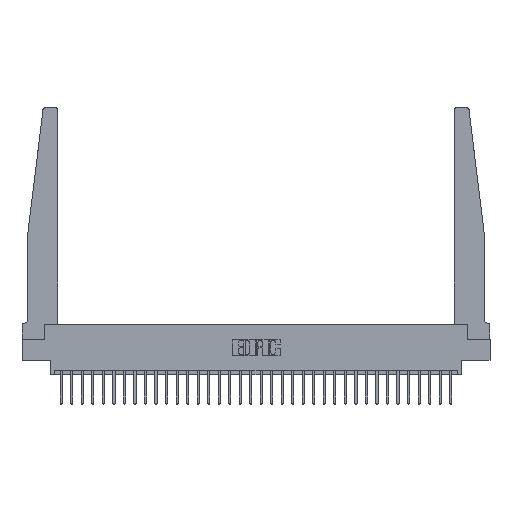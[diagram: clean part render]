
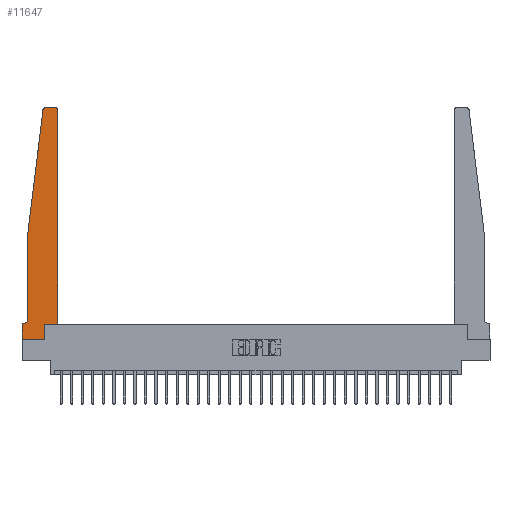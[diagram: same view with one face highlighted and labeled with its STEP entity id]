
A CAD part, top view. The second image highlights one B-rep face of the part: STEP entity #11647.
In plain terms, the highlighted planar face has unit normal (0, 0, 1).
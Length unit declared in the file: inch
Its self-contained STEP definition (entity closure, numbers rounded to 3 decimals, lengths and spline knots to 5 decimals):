
#126 = FACE_OUTER_BOUND ( 'NONE', #1738, .T. ) ;
#573 = DIRECTION ( 'NONE',  ( 1., 0., 0. ) ) ;
#765 = DIRECTION ( 'NONE',  ( -1., 0., 0. ) ) ;
#1738 = EDGE_LOOP ( 'NONE', ( #14604, #15511, #18956, #3326, #2910, #1840, #23805, #4217, #19365, #21651, #21464, #3063 ) ) ;
#1840 = ORIENTED_EDGE ( 'NONE', *, *, #16754, .T. ) ;
#2118 = CARTESIAN_POINT ( 'NONE',  ( 0.25, 2.75, 0.37 ) ) ;
#2347 = VECTOR ( 'NONE', #26820, 39.37008 ) ;
#2727 = VECTOR ( 'NONE', #13173, 39.37008 ) ;
#2849 = VERTEX_POINT ( 'NONE', #7482 ) ;
#2910 = ORIENTED_EDGE ( 'NONE', *, *, #19594, .T. ) ;
#3063 = ORIENTED_EDGE ( 'NONE', *, *, #20286, .T. ) ;
#3131 = VERTEX_POINT ( 'NONE', #7297 ) ;
#3290 = CARTESIAN_POINT ( 'NONE',  ( 0., 0., 0.37 ) ) ;
#3326 = ORIENTED_EDGE ( 'NONE', *, *, #26223, .T. ) ;
#3501 = VERTEX_POINT ( 'NONE', #27071 ) ;
#3511 = VECTOR ( 'NONE', #28980, 39.37008 ) ;
#3869 = DIRECTION ( 'NONE',  ( 1., 0., 0. ) ) ;
#4111 = LINE ( 'NONE', #18639, #15181 ) ;
#4217 = ORIENTED_EDGE ( 'NONE', *, *, #26971, .T. ) ;
#4443 = LINE ( 'NONE', #2118, #30245 ) ;
#5444 = CARTESIAN_POINT ( 'NONE',  ( 0.27653, 2.75, 0.37 ) ) ;
#5943 = LINE ( 'NONE', #15333, #2347 ) ;
#6011 = VERTEX_POINT ( 'NONE', #18988 ) ;
#7297 = CARTESIAN_POINT ( 'NONE',  ( 0.425, 0.18, 0.37 ) ) ;
#7482 = CARTESIAN_POINT ( 'NONE',  ( 0.2605, 0.18, 0.37 ) ) ;
#9328 = CARTESIAN_POINT ( 'NONE',  ( 0., 0.1875, 0.37 ) ) ;
#9490 = CARTESIAN_POINT ( 'NONE',  ( 0., 0.1875, 0.37 ) ) ;
#9556 = CIRCLE ( 'NONE', #13543, 0.03 ) ;
#9811 = LINE ( 'NONE', #11715, #11964 ) ;
#10346 = LINE ( 'NONE', #25306, #2727 ) ;
#10511 = DIRECTION ( 'NONE',  ( 1., 0., 0. ) ) ;
#10516 = VERTEX_POINT ( 'NONE', #26833 ) ;
#11459 = EDGE_CURVE ( 'NONE', #6011, #2849, #19803, .T. ) ;
#11647 = ADVANCED_FACE ( 'NONE', ( #126 ), #14461, .T. ) ;
#11715 = CARTESIAN_POINT ( 'NONE',  ( 0.065, 1.25, 0.37 ) ) ;
#11759 = VECTOR ( 'NONE', #573, 39.37008 ) ;
#11964 = VECTOR ( 'NONE', #23856, 39.37008 ) ;
#12364 = LINE ( 'NONE', #19540, #3511 ) ;
#12996 = VERTEX_POINT ( 'NONE', #14139 ) ;
#13173 = DIRECTION ( 'NONE',  ( 0., -1., 0. ) ) ;
#13422 = EDGE_CURVE ( 'NONE', #3131, #24890, #4111, .T. ) ;
#13543 = AXIS2_PLACEMENT_3D ( 'NONE', #29840, #24900, #3869 ) ;
#13636 = DIRECTION ( 'NONE',  ( 0., 1., 0. ) ) ;
#14139 = CARTESIAN_POINT ( 'NONE',  ( 0.395, 2.75, 0.37 ) ) ;
#14255 = AXIS2_PLACEMENT_3D ( 'NONE', #22997, #15521, #10511 ) ;
#14461 = PLANE ( 'NONE',  #19592 ) ;
#14604 = ORIENTED_EDGE ( 'NONE', *, *, #30408, .T. ) ;
#14779 = LINE ( 'NONE', #17417, #11759 ) ;
#14831 = EDGE_CURVE ( 'NONE', #21649, #27962, #5943, .T. ) ;
#15181 = VECTOR ( 'NONE', #13636, 39.37008 ) ;
#15333 = CARTESIAN_POINT ( 'NONE',  ( 0., 0., 0.37 ) ) ;
#15511 = ORIENTED_EDGE ( 'NONE', *, *, #27499, .T. ) ;
#15521 = DIRECTION ( 'NONE',  ( 0., 0., 1. ) ) ;
#16754 = EDGE_CURVE ( 'NONE', #3501, #21649, #17145, .T. ) ;
#17145 = LINE ( 'NONE', #21131, #18878 ) ;
#17417 = CARTESIAN_POINT ( 'NONE',  ( 0., 0., 0.37 ) ) ;
#18247 = CIRCLE ( 'NONE', #14255, 0.03 ) ;
#18352 = VERTEX_POINT ( 'NONE', #23576 ) ;
#18365 = EDGE_CURVE ( 'NONE', #10516, #26652, #9811, .T. ) ;
#18639 = CARTESIAN_POINT ( 'NONE',  ( 0.425, 0.18, 0.37 ) ) ;
#18848 = DIRECTION ( 'NONE',  ( 1., 0., 0. ) ) ;
#18878 = VECTOR ( 'NONE', #765, 39.37008 ) ;
#18902 = CARTESIAN_POINT ( 'NONE',  ( 0.015, 0.2375, 0.37 ) ) ;
#18956 = ORIENTED_EDGE ( 'NONE', *, *, #18365, .T. ) ;
#18988 = CARTESIAN_POINT ( 'NONE',  ( 0.2605, 0., 0.37 ) ) ;
#19047 = DIRECTION ( 'NONE',  ( -1., 0., 0. ) ) ;
#19097 = VECTOR ( 'NONE', #19956, 39.37008 ) ;
#19213 = EDGE_CURVE ( 'NONE', #2849, #3131, #12364, .T. ) ;
#19365 = ORIENTED_EDGE ( 'NONE', *, *, #11459, .T. ) ;
#19540 = CARTESIAN_POINT ( 'NONE',  ( 0.425, 0.18, 0.37 ) ) ;
#19592 = AXIS2_PLACEMENT_3D ( 'NONE', #9328, #25684, #18848 ) ;
#19594 = EDGE_CURVE ( 'NONE', #18352, #3501, #20472, .T. ) ;
#19803 = LINE ( 'NONE', #22147, #19097 ) ;
#19956 = DIRECTION ( 'NONE',  ( 0., 1., 0. ) ) ;
#20286 = EDGE_CURVE ( 'NONE', #24890, #12996, #9556, .T. ) ;
#20472 = CIRCLE ( 'NONE', #24425, 0.05 ) ;
#21131 = CARTESIAN_POINT ( 'NONE',  ( 0.065, 0.1875, 0.37 ) ) ;
#21158 = DIRECTION ( 'NONE',  ( -1., 0., 0. ) ) ;
#21464 = ORIENTED_EDGE ( 'NONE', *, *, #13422, .T. ) ;
#21649 = VERTEX_POINT ( 'NONE', #9490 ) ;
#21651 = ORIENTED_EDGE ( 'NONE', *, *, #19213, .T. ) ;
#22147 = CARTESIAN_POINT ( 'NONE',  ( 0.2605, 0.18, 0.37 ) ) ;
#22997 = CARTESIAN_POINT ( 'NONE',  ( 0.27653, 2.72, 0.37 ) ) ;
#23576 = CARTESIAN_POINT ( 'NONE',  ( 0.065, 0.2375, 0.37 ) ) ;
#23805 = ORIENTED_EDGE ( 'NONE', *, *, #14831, .T. ) ;
#23856 = DIRECTION ( 'NONE',  ( -0.122, -0.992, 0. ) ) ;
#24425 = AXIS2_PLACEMENT_3D ( 'NONE', #18902, #28780, #19047 ) ;
#24890 = VERTEX_POINT ( 'NONE', #26015 ) ;
#24900 = DIRECTION ( 'NONE',  ( 0., 0., 1. ) ) ;
#25306 = CARTESIAN_POINT ( 'NONE',  ( 0.065, 1.25, 0.37 ) ) ;
#25542 = CARTESIAN_POINT ( 'NONE',  ( 0.065, 1.25, 0.37 ) ) ;
#25684 = DIRECTION ( 'NONE',  ( 0., 0., 1. ) ) ;
#26015 = CARTESIAN_POINT ( 'NONE',  ( 0.425, 2.72, 0.37 ) ) ;
#26223 = EDGE_CURVE ( 'NONE', #26652, #18352, #10346, .T. ) ;
#26652 = VERTEX_POINT ( 'NONE', #25542 ) ;
#26820 = DIRECTION ( 'NONE',  ( 0., -1., 0. ) ) ;
#26833 = CARTESIAN_POINT ( 'NONE',  ( 0.24675, 2.72367, 0.37 ) ) ;
#26971 = EDGE_CURVE ( 'NONE', #27962, #6011, #14779, .T. ) ;
#27071 = CARTESIAN_POINT ( 'NONE',  ( 0.015, 0.1875, 0.37 ) ) ;
#27499 = EDGE_CURVE ( 'NONE', #28384, #10516, #18247, .T. ) ;
#27962 = VERTEX_POINT ( 'NONE', #3290 ) ;
#28384 = VERTEX_POINT ( 'NONE', #5444 ) ;
#28780 = DIRECTION ( 'NONE',  ( 0., 0., -1. ) ) ;
#28980 = DIRECTION ( 'NONE',  ( 1., 0., 0. ) ) ;
#29840 = CARTESIAN_POINT ( 'NONE',  ( 0.395, 2.72, 0.37 ) ) ;
#30245 = VECTOR ( 'NONE', #21158, 39.37008 ) ;
#30408 = EDGE_CURVE ( 'NONE', #12996, #28384, #4443, .T. ) ;
